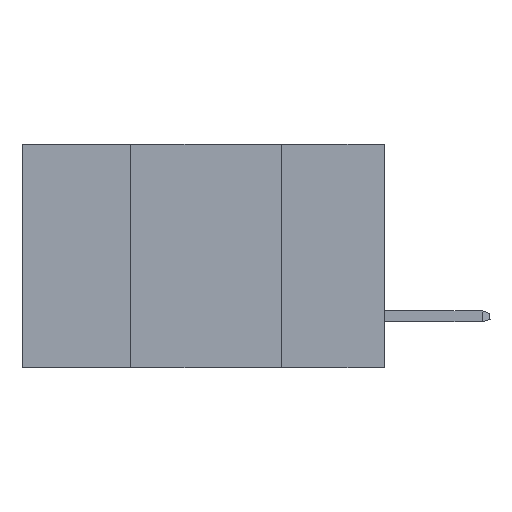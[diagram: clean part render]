
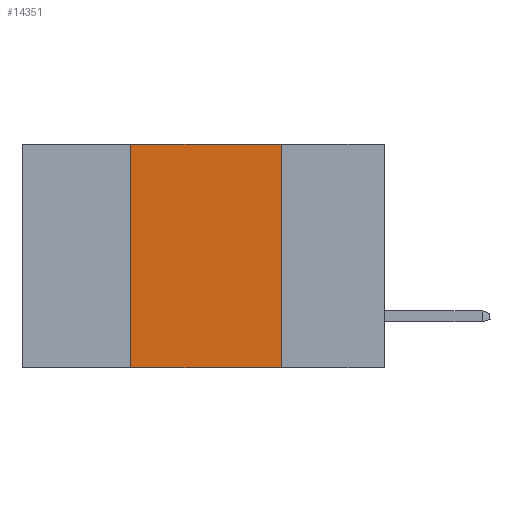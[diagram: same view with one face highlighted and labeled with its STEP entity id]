
A CAD part, left-side view. The second image highlights one B-rep face of the part: STEP entity #14351.
In plain terms, the highlighted planar face has unit normal (-1, 0, 0).
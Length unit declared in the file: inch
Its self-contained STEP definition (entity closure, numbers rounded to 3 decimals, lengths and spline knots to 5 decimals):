
#42 = CARTESIAN_POINT ( 'NONE',  ( 0., 0.6, -0.37 ) ) ;
#193 = ORIENTED_EDGE ( 'NONE', *, *, #20171, .F. ) ;
#212 = EDGE_CURVE ( 'NONE', #9196, #1163, #25894, .T. ) ;
#798 = EDGE_LOOP ( 'NONE', ( #193, #20413, #9313, #24421 ) ) ;
#1163 = VERTEX_POINT ( 'NONE', #23059 ) ;
#1469 = LINE ( 'NONE', #6444, #26712 ) ;
#2555 = VERTEX_POINT ( 'NONE', #8506 ) ;
#6390 = DIRECTION ( 'NONE',  ( 1., 0., 0. ) ) ;
#6444 = CARTESIAN_POINT ( 'NONE',  ( 0., 0.17, 0. ) ) ;
#7331 = CARTESIAN_POINT ( 'NONE',  ( 0., 0.6, 0. ) ) ;
#7350 = FACE_OUTER_BOUND ( 'NONE', #798, .T. ) ;
#7847 = DIRECTION ( 'NONE',  ( 0., 0., 1. ) ) ;
#8506 = CARTESIAN_POINT ( 'NONE',  ( 0., 0.42, 0. ) ) ;
#9196 = VERTEX_POINT ( 'NONE', #22944 ) ;
#9313 = ORIENTED_EDGE ( 'NONE', *, *, #14093, .F. ) ;
#10578 = LINE ( 'NONE', #7331, #26641 ) ;
#10651 = DIRECTION ( 'NONE',  ( 0., 0., -1. ) ) ;
#10788 = CARTESIAN_POINT ( 'NONE',  ( 0., 0.6, 0. ) ) ;
#11958 = CARTESIAN_POINT ( 'NONE',  ( 0., 0.42, 0. ) ) ;
#14093 = EDGE_CURVE ( 'NONE', #9196, #2555, #17544, .T. ) ;
#14351 = ADVANCED_FACE ( 'NONE', ( #7350 ), #14571, .F. ) ;
#14571 = PLANE ( 'NONE',  #20572 ) ;
#15248 = CARTESIAN_POINT ( 'NONE',  ( 0., 0.17, 0. ) ) ;
#15302 = EDGE_CURVE ( 'NONE', #2555, #20847, #10578, .T. ) ;
#17544 = LINE ( 'NONE', #11958, #18534 ) ;
#18534 = VECTOR ( 'NONE', #7847, 39.37008 ) ;
#19210 = DIRECTION ( 'NONE',  ( 0., -1., 0. ) ) ;
#20171 = EDGE_CURVE ( 'NONE', #20847, #1163, #1469, .T. ) ;
#20413 = ORIENTED_EDGE ( 'NONE', *, *, #15302, .F. ) ;
#20572 = AXIS2_PLACEMENT_3D ( 'NONE', #10788, #6390, #21079 ) ;
#20847 = VERTEX_POINT ( 'NONE', #15248 ) ;
#21079 = DIRECTION ( 'NONE',  ( 0., 0., -1. ) ) ;
#22944 = CARTESIAN_POINT ( 'NONE',  ( 0., 0.42, -0.37 ) ) ;
#23059 = CARTESIAN_POINT ( 'NONE',  ( 0., 0.17, -0.37 ) ) ;
#24421 = ORIENTED_EDGE ( 'NONE', *, *, #212, .T. ) ;
#25247 = VECTOR ( 'NONE', #19210, 39.37008 ) ;
#25894 = LINE ( 'NONE', #42, #25247 ) ;
#26641 = VECTOR ( 'NONE', #27090, 39.37008 ) ;
#26712 = VECTOR ( 'NONE', #10651, 39.37008 ) ;
#27090 = DIRECTION ( 'NONE',  ( 0., -1., 0. ) ) ;
